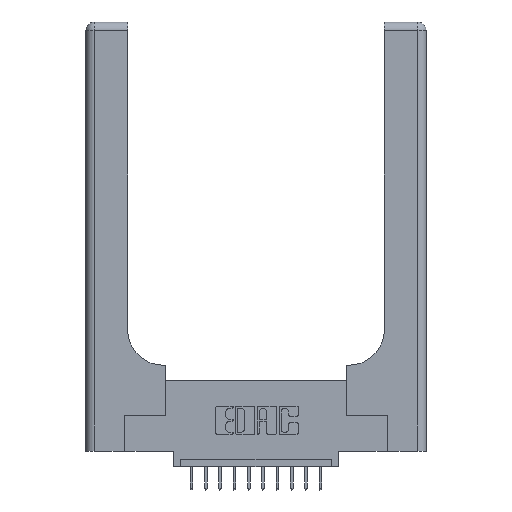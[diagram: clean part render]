
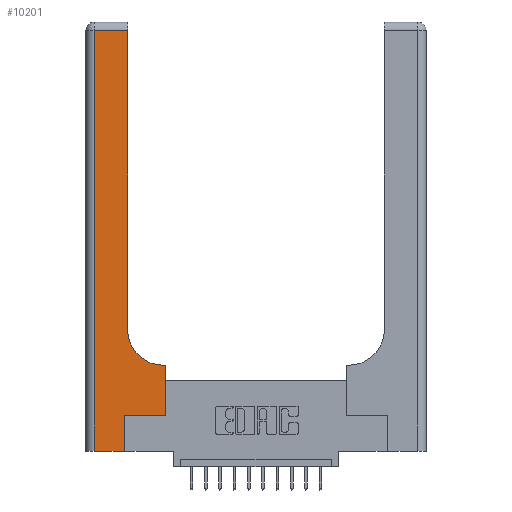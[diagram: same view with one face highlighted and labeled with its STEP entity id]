
A CAD part, top view. The second image highlights one B-rep face of the part: STEP entity #10201.
In plain terms, the highlighted planar face has unit normal (0, 0, 1).
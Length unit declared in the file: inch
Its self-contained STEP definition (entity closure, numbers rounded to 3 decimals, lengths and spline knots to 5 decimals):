
#232 = VERTEX_POINT ( 'NONE', #1740 ) ;
#527 = DIRECTION ( 'NONE',  ( -1., 0., 0. ) ) ;
#541 = CARTESIAN_POINT ( 'NONE',  ( 0.5415, 0.6, 0.37 ) ) ;
#637 = ORIENTED_EDGE ( 'NONE', *, *, #5552, .T. ) ;
#1383 = VERTEX_POINT ( 'NONE', #5928 ) ;
#1490 = DIRECTION ( 'NONE',  ( 0., 1., 0. ) ) ;
#1540 = ORIENTED_EDGE ( 'NONE', *, *, #6683, .T. ) ;
#1740 = CARTESIAN_POINT ( 'NONE',  ( 0.06, 0., 0.37 ) ) ;
#1863 = CARTESIAN_POINT ( 'NONE',  ( 0., 2.94, 0.37 ) ) ;
#2111 = LINE ( 'NONE', #1863, #10438 ) ;
#2141 = DIRECTION ( 'NONE',  ( 0., 0., -1. ) ) ;
#2348 = ORIENTED_EDGE ( 'NONE', *, *, #2603, .T. ) ;
#2603 = EDGE_CURVE ( 'NONE', #15660, #3588, #11555, .T. ) ;
#2621 = CARTESIAN_POINT ( 'NONE',  ( 0.2915, 0.85, 0.37 ) ) ;
#2967 = VECTOR ( 'NONE', #7503, 39.37008 ) ;
#3134 = VERTEX_POINT ( 'NONE', #7930 ) ;
#3180 = CARTESIAN_POINT ( 'NONE',  ( 0.269, 0., 0.37 ) ) ;
#3588 = VERTEX_POINT ( 'NONE', #9348 ) ;
#3708 = EDGE_CURVE ( 'NONE', #3588, #6572, #14454, .T. ) ;
#3927 = ORIENTED_EDGE ( 'NONE', *, *, #6809, .T. ) ;
#4084 = VECTOR ( 'NONE', #1490, 39.37008 ) ;
#4195 = VECTOR ( 'NONE', #9763, 39.37008 ) ;
#4405 = AXIS2_PLACEMENT_3D ( 'NONE', #7015, #2141, #16897 ) ;
#4863 = CARTESIAN_POINT ( 'NONE',  ( 0.2915, 3., 0.37 ) ) ;
#5160 = CARTESIAN_POINT ( 'NONE',  ( 0., 3., 0.37 ) ) ;
#5290 = EDGE_CURVE ( 'NONE', #14575, #3134, #2111, .T. ) ;
#5311 = EDGE_CURVE ( 'NONE', #1383, #15660, #14388, .T. ) ;
#5408 = CARTESIAN_POINT ( 'NONE',  ( 0.5585, 0.25, 0.37 ) ) ;
#5426 = CARTESIAN_POINT ( 'NONE',  ( 0.5585, 0.25, 0.37 ) ) ;
#5481 = DIRECTION ( 'NONE',  ( -1., 0., 0. ) ) ;
#5552 = EDGE_CURVE ( 'NONE', #8036, #1383, #6259, .T. ) ;
#5928 = CARTESIAN_POINT ( 'NONE',  ( 0.269, 0.25, 0.37 ) ) ;
#6100 = VECTOR ( 'NONE', #10176, 39.37008 ) ;
#6207 = AXIS2_PLACEMENT_3D ( 'NONE', #5160, #15928, #9118 ) ;
#6259 = LINE ( 'NONE', #3180, #16887 ) ;
#6489 = LINE ( 'NONE', #16589, #2967 ) ;
#6572 = VERTEX_POINT ( 'NONE', #541 ) ;
#6683 = EDGE_CURVE ( 'NONE', #3134, #232, #10191, .T. ) ;
#6809 = EDGE_CURVE ( 'NONE', #6572, #9323, #9358, .T. ) ;
#6898 = CARTESIAN_POINT ( 'NONE',  ( 0.269, 0., 0.37 ) ) ;
#7015 = CARTESIAN_POINT ( 'NONE',  ( 0.5415, 0.85, 0.37 ) ) ;
#7503 = DIRECTION ( 'NONE',  ( 1., 0., 0. ) ) ;
#7711 = PLANE ( 'NONE',  #6207 ) ;
#7930 = CARTESIAN_POINT ( 'NONE',  ( 0.06, 2.94, 0.37 ) ) ;
#8036 = VERTEX_POINT ( 'NONE', #6898 ) ;
#8184 = ORIENTED_EDGE ( 'NONE', *, *, #3708, .T. ) ;
#8555 = ORIENTED_EDGE ( 'NONE', *, *, #5311, .T. ) ;
#8581 = DIRECTION ( 'NONE',  ( 0., 1., 0. ) ) ;
#9000 = DIRECTION ( 'NONE',  ( 0., -1., 0. ) ) ;
#9118 = DIRECTION ( 'NONE',  ( -1., 0., 0. ) ) ;
#9323 = VERTEX_POINT ( 'NONE', #2621 ) ;
#9348 = CARTESIAN_POINT ( 'NONE',  ( 0.5585, 0.6, 0.37 ) ) ;
#9358 = CIRCLE ( 'NONE', #4405, 0.25 ) ;
#9763 = DIRECTION ( 'NONE',  ( 1., 0., 0. ) ) ;
#9786 = ORIENTED_EDGE ( 'NONE', *, *, #12716, .T. ) ;
#10176 = DIRECTION ( 'NONE',  ( 0., 1., 0. ) ) ;
#10191 = LINE ( 'NONE', #15534, #16842 ) ;
#10201 = ADVANCED_FACE ( 'NONE', ( #15585 ), #7711, .F. ) ;
#10438 = VECTOR ( 'NONE', #527, 39.37008 ) ;
#11517 = LINE ( 'NONE', #4863, #6100 ) ;
#11555 = LINE ( 'NONE', #5426, #4084 ) ;
#12716 = EDGE_CURVE ( 'NONE', #9323, #14575, #11517, .T. ) ;
#12996 = CARTESIAN_POINT ( 'NONE',  ( 0.2915, 2.94, 0.37 ) ) ;
#14033 = ORIENTED_EDGE ( 'NONE', *, *, #16950, .T. ) ;
#14375 = EDGE_LOOP ( 'NONE', ( #9786, #15788, #1540, #14033, #637, #8555, #2348, #8184, #3927 ) ) ;
#14388 = LINE ( 'NONE', #15178, #4195 ) ;
#14454 = LINE ( 'NONE', #16073, #17149 ) ;
#14575 = VERTEX_POINT ( 'NONE', #12996 ) ;
#15178 = CARTESIAN_POINT ( 'NONE',  ( 0.269, 0.25, 0.37 ) ) ;
#15534 = CARTESIAN_POINT ( 'NONE',  ( 0.06, 3., 0.37 ) ) ;
#15585 = FACE_OUTER_BOUND ( 'NONE', #14375, .T. ) ;
#15660 = VERTEX_POINT ( 'NONE', #5408 ) ;
#15788 = ORIENTED_EDGE ( 'NONE', *, *, #5290, .T. ) ;
#15928 = DIRECTION ( 'NONE',  ( 0., 0., -1. ) ) ;
#16073 = CARTESIAN_POINT ( 'NONE',  ( 0.2915, 0.6, 0.37 ) ) ;
#16589 = CARTESIAN_POINT ( 'NONE',  ( 0., 0., 0.37 ) ) ;
#16842 = VECTOR ( 'NONE', #9000, 39.37008 ) ;
#16887 = VECTOR ( 'NONE', #8581, 39.37008 ) ;
#16897 = DIRECTION ( 'NONE',  ( 1., 0., 0. ) ) ;
#16950 = EDGE_CURVE ( 'NONE', #232, #8036, #6489, .T. ) ;
#17149 = VECTOR ( 'NONE', #5481, 39.37008 ) ;
